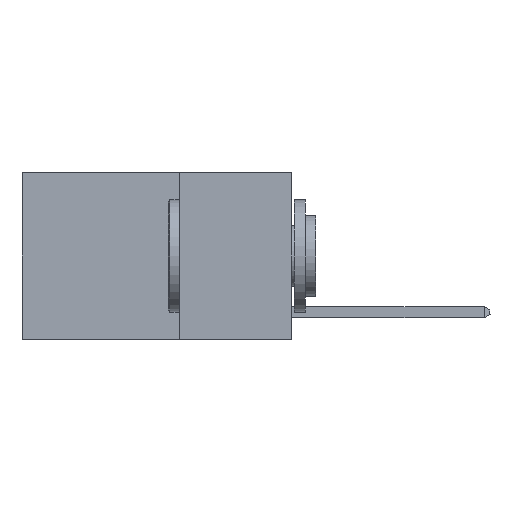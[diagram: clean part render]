
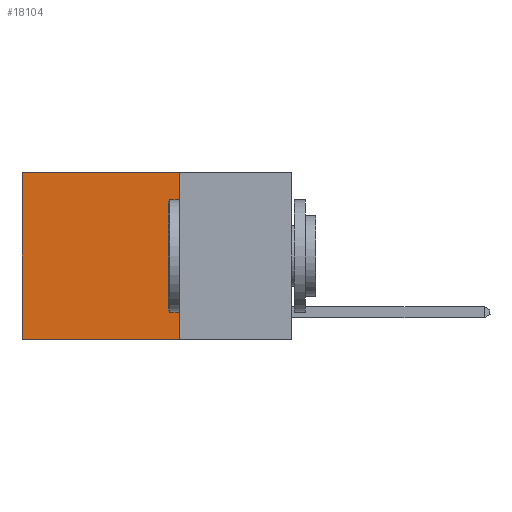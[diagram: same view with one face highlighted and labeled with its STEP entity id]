
A CAD part, left-side view. The second image highlights one B-rep face of the part: STEP entity #18104.
In plain terms, the highlighted planar face has unit normal (-1, 0, 0).
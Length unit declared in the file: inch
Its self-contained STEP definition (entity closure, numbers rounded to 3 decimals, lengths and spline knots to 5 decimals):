
#629 = LINE ( 'NONE', #13796, #7066 ) ;
#1779 = VECTOR ( 'NONE', #19683, 39.37008 ) ;
#2074 = VERTEX_POINT ( 'NONE', #11801 ) ;
#2617 = VERTEX_POINT ( 'NONE', #20271 ) ;
#3750 = CARTESIAN_POINT ( 'NONE',  ( 0.2625, 0.25, 0. ) ) ;
#5185 = EDGE_CURVE ( 'NONE', #6224, #9370, #629, .T. ) ;
#5896 = DIRECTION ( 'NONE',  ( 0., 0., -1. ) ) ;
#5961 = EDGE_LOOP ( 'NONE', ( #13648, #16939, #11042, #20463 ) ) ;
#6224 = VERTEX_POINT ( 'NONE', #18975 ) ;
#7065 = DIRECTION ( 'NONE',  ( 0., 1., 0. ) ) ;
#7066 = VECTOR ( 'NONE', #7065, 39.37008 ) ;
#8197 = EDGE_CURVE ( 'NONE', #6224, #2074, #16619, .T. ) ;
#8660 = VECTOR ( 'NONE', #12666, 39.37008 ) ;
#8855 = VECTOR ( 'NONE', #10991, 39.37008 ) ;
#9051 = EDGE_CURVE ( 'NONE', #2074, #2617, #20473, .T. ) ;
#9170 = PLANE ( 'NONE',  #19356 ) ;
#9370 = VERTEX_POINT ( 'NONE', #13513 ) ;
#10991 = DIRECTION ( 'NONE',  ( 0., 1., 0. ) ) ;
#11042 = ORIENTED_EDGE ( 'NONE', *, *, #8197, .F. ) ;
#11801 = CARTESIAN_POINT ( 'NONE',  ( 0.2625, 0.25, -0.37 ) ) ;
#12666 = DIRECTION ( 'NONE',  ( 0., 0., -1. ) ) ;
#13513 = CARTESIAN_POINT ( 'NONE',  ( 0.2625, 0.6, 0. ) ) ;
#13648 = ORIENTED_EDGE ( 'NONE', *, *, #13678, .T. ) ;
#13678 = EDGE_CURVE ( 'NONE', #9370, #2617, #17722, .T. ) ;
#13796 = CARTESIAN_POINT ( 'NONE',  ( 0.2625, 0.25, 0. ) ) ;
#14233 = CARTESIAN_POINT ( 'NONE',  ( 0.2625, 0.6, 0. ) ) ;
#14245 = CARTESIAN_POINT ( 'NONE',  ( 0.2625, 0.25, -0.37 ) ) ;
#15473 = CARTESIAN_POINT ( 'NONE',  ( 0.2625, 0.25, 0. ) ) ;
#16619 = LINE ( 'NONE', #3750, #1779 ) ;
#16939 = ORIENTED_EDGE ( 'NONE', *, *, #9051, .F. ) ;
#17594 = FACE_OUTER_BOUND ( 'NONE', #5961, .T. ) ;
#17722 = LINE ( 'NONE', #14233, #8660 ) ;
#18104 = ADVANCED_FACE ( 'NONE', ( #17594 ), #9170, .F. ) ;
#18975 = CARTESIAN_POINT ( 'NONE',  ( 0.2625, 0.25, 0. ) ) ;
#19356 = AXIS2_PLACEMENT_3D ( 'NONE', #15473, #20340, #5896 ) ;
#19683 = DIRECTION ( 'NONE',  ( 0., 0., -1. ) ) ;
#20271 = CARTESIAN_POINT ( 'NONE',  ( 0.2625, 0.6, -0.37 ) ) ;
#20340 = DIRECTION ( 'NONE',  ( 1., 0., 0. ) ) ;
#20463 = ORIENTED_EDGE ( 'NONE', *, *, #5185, .T. ) ;
#20473 = LINE ( 'NONE', #14245, #8855 ) ;
